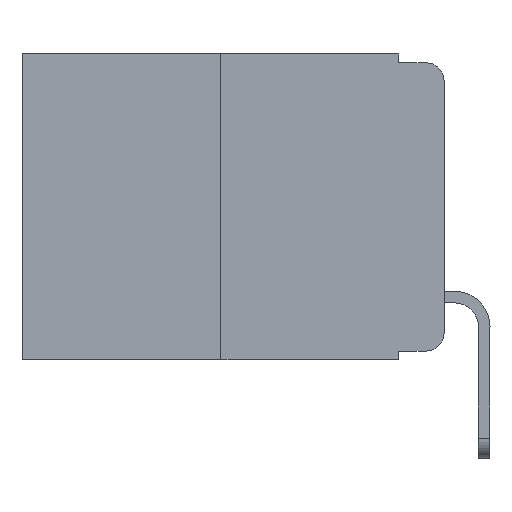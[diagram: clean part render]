
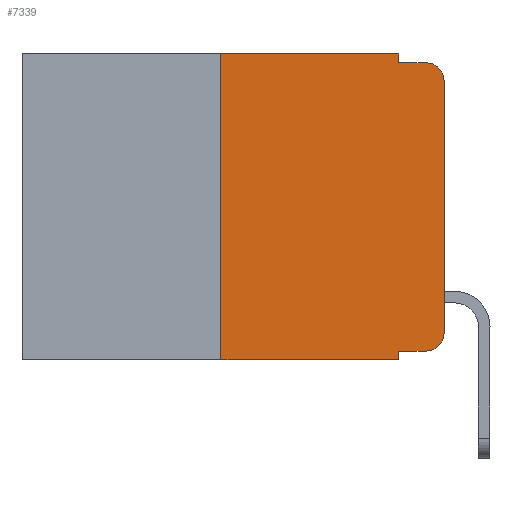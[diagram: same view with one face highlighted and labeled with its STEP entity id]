
A CAD part, left-side view. The second image highlights one B-rep face of the part: STEP entity #7339.
In plain terms, the highlighted planar face has unit normal (-1, 0, 0).
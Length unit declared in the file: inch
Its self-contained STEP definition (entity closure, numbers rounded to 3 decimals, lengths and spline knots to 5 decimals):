
#1022 = EDGE_CURVE ( 'NONE', #13276, #21223, #18763, .T. ) ;
#1138 = VECTOR ( 'NONE', #13843, 39.37008 ) ;
#1317 = AXIS2_PLACEMENT_3D ( 'NONE', #7727, #9491, #21742 ) ;
#1612 = CARTESIAN_POINT ( 'NONE',  ( 0., 0.051, -0.01 ) ) ;
#1954 = EDGE_CURVE ( 'NONE', #13807, #6931, #13780, .T. ) ;
#2329 = CARTESIAN_POINT ( 'NONE',  ( 0., 0.051, 0. ) ) ;
#2383 = ORIENTED_EDGE ( 'NONE', *, *, #6162, .T. ) ;
#2544 = CARTESIAN_POINT ( 'NONE',  ( 0., 0.473, 0. ) ) ;
#2577 = ORIENTED_EDGE ( 'NONE', *, *, #4874, .F. ) ;
#3516 = LINE ( 'NONE', #19200, #16099 ) ;
#4874 = EDGE_CURVE ( 'NONE', #8076, #8535, #6316, .T. ) ;
#5457 = CARTESIAN_POINT ( 'NONE',  ( 0., 0.02, -0.333 ) ) ;
#5822 = DIRECTION ( 'NONE',  ( 0., 0., 1. ) ) ;
#5853 = DIRECTION ( 'NONE',  ( 0., 0., -1. ) ) ;
#5892 = VECTOR ( 'NONE', #15665, 39.37008 ) ;
#5964 = AXIS2_PLACEMENT_3D ( 'NONE', #21284, #9038, #14331 ) ;
#6004 = VECTOR ( 'NONE', #15671, 39.37008 ) ;
#6162 = EDGE_CURVE ( 'NONE', #13807, #6469, #3516, .T. ) ;
#6282 = ORIENTED_EDGE ( 'NONE', *, *, #1954, .F. ) ;
#6316 = LINE ( 'NONE', #1612, #1138 ) ;
#6362 = CARTESIAN_POINT ( 'NONE',  ( 0., 0.473, 0. ) ) ;
#6446 = EDGE_CURVE ( 'NONE', #6931, #14911, #11437, .T. ) ;
#6469 = VERTEX_POINT ( 'NONE', #14853 ) ;
#6848 = DIRECTION ( 'NONE',  ( 0., -1., 0. ) ) ;
#6931 = VERTEX_POINT ( 'NONE', #18444 ) ;
#7141 = EDGE_CURVE ( 'NONE', #20674, #8535, #19628, .T. ) ;
#7339 = ADVANCED_FACE ( 'NONE', ( #20976 ), #18306, .F. ) ;
#7727 = CARTESIAN_POINT ( 'NONE',  ( 0., 0.02, -0.313 ) ) ;
#8076 = VERTEX_POINT ( 'NONE', #15927 ) ;
#8535 = VERTEX_POINT ( 'NONE', #22609 ) ;
#8542 = EDGE_CURVE ( 'NONE', #11496, #20674, #19854, .T. ) ;
#9038 = DIRECTION ( 'NONE',  ( -1., 0., 0. ) ) ;
#9491 = DIRECTION ( 'NONE',  ( -1., 0., 0. ) ) ;
#9571 = DIRECTION ( 'NONE',  ( 0., -1., 0. ) ) ;
#10452 = CARTESIAN_POINT ( 'NONE',  ( 0., 0.051, 0. ) ) ;
#11008 = CARTESIAN_POINT ( 'NONE',  ( 0., 0.25, 0. ) ) ;
#11169 = VECTOR ( 'NONE', #9571, 39.37008 ) ;
#11437 = LINE ( 'NONE', #2544, #11169 ) ;
#11496 = VERTEX_POINT ( 'NONE', #19450 ) ;
#12102 = ORIENTED_EDGE ( 'NONE', *, *, #7141, .T. ) ;
#12512 = ORIENTED_EDGE ( 'NONE', *, *, #19481, .T. ) ;
#12535 = CARTESIAN_POINT ( 'NONE',  ( 0., 0.051, 0. ) ) ;
#12681 = CARTESIAN_POINT ( 'NONE',  ( 0., 0., -0.03 ) ) ;
#13096 = EDGE_LOOP ( 'NONE', ( #14808, #12102, #2577, #18624, #14434, #6282, #2383, #19252, #14275, #12512 ) ) ;
#13276 = VERTEX_POINT ( 'NONE', #13291 ) ;
#13291 = CARTESIAN_POINT ( 'NONE',  ( 0., 0.051, -0.333 ) ) ;
#13780 = LINE ( 'NONE', #11008, #18166 ) ;
#13807 = VERTEX_POINT ( 'NONE', #19998 ) ;
#13843 = DIRECTION ( 'NONE',  ( 0., -1., 0. ) ) ;
#13905 = CARTESIAN_POINT ( 'NONE',  ( 0., 0., 0. ) ) ;
#14275 = ORIENTED_EDGE ( 'NONE', *, *, #1022, .T. ) ;
#14331 = DIRECTION ( 'NONE',  ( 0., 0., -1. ) ) ;
#14434 = ORIENTED_EDGE ( 'NONE', *, *, #6446, .F. ) ;
#14808 = ORIENTED_EDGE ( 'NONE', *, *, #8542, .T. ) ;
#14853 = CARTESIAN_POINT ( 'NONE',  ( 0., 0.051, -0.343 ) ) ;
#14900 = AXIS2_PLACEMENT_3D ( 'NONE', #6362, #16689, #18535 ) ;
#14911 = VERTEX_POINT ( 'NONE', #12535 ) ;
#15028 = LINE ( 'NONE', #10452, #6004 ) ;
#15340 = CARTESIAN_POINT ( 'NONE',  ( 0., 0.051, -0.333 ) ) ;
#15665 = DIRECTION ( 'NONE',  ( 0., 0., 1. ) ) ;
#15671 = DIRECTION ( 'NONE',  ( 0., 0., -1. ) ) ;
#15927 = CARTESIAN_POINT ( 'NONE',  ( 0., 0.051, -0.01 ) ) ;
#16099 = VECTOR ( 'NONE', #19049, 39.37008 ) ;
#16527 = EDGE_CURVE ( 'NONE', #13276, #6469, #15028, .T. ) ;
#16689 = DIRECTION ( 'NONE',  ( 1., 0., 0. ) ) ;
#17480 = EDGE_CURVE ( 'NONE', #14911, #8076, #22338, .T. ) ;
#18165 = CIRCLE ( 'NONE', #1317, 0.02 ) ;
#18166 = VECTOR ( 'NONE', #5822, 39.37008 ) ;
#18306 = PLANE ( 'NONE',  #14900 ) ;
#18444 = CARTESIAN_POINT ( 'NONE',  ( 0., 0.25, 0. ) ) ;
#18535 = DIRECTION ( 'NONE',  ( 0., 0., -1. ) ) ;
#18624 = ORIENTED_EDGE ( 'NONE', *, *, #17480, .F. ) ;
#18763 = LINE ( 'NONE', #15340, #21755 ) ;
#19049 = DIRECTION ( 'NONE',  ( 0., -1., 0. ) ) ;
#19200 = CARTESIAN_POINT ( 'NONE',  ( 0., 0.473, -0.343 ) ) ;
#19252 = ORIENTED_EDGE ( 'NONE', *, *, #16527, .F. ) ;
#19366 = VECTOR ( 'NONE', #5853, 39.37008 ) ;
#19450 = CARTESIAN_POINT ( 'NONE',  ( 0., 0., -0.313 ) ) ;
#19481 = EDGE_CURVE ( 'NONE', #21223, #11496, #18165, .T. ) ;
#19628 = CIRCLE ( 'NONE', #5964, 0.02 ) ;
#19854 = LINE ( 'NONE', #13905, #5892 ) ;
#19998 = CARTESIAN_POINT ( 'NONE',  ( 0., 0.25, -0.343 ) ) ;
#20674 = VERTEX_POINT ( 'NONE', #12681 ) ;
#20976 = FACE_OUTER_BOUND ( 'NONE', #13096, .T. ) ;
#21223 = VERTEX_POINT ( 'NONE', #5457 ) ;
#21284 = CARTESIAN_POINT ( 'NONE',  ( 0., 0.02, -0.03 ) ) ;
#21742 = DIRECTION ( 'NONE',  ( 0., 0., -1. ) ) ;
#21755 = VECTOR ( 'NONE', #6848, 39.37008 ) ;
#22338 = LINE ( 'NONE', #2329, #19366 ) ;
#22609 = CARTESIAN_POINT ( 'NONE',  ( 0., 0.02, -0.01 ) ) ;
